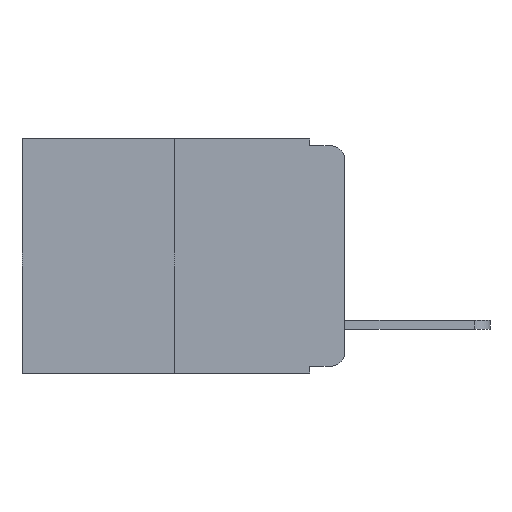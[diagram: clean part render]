
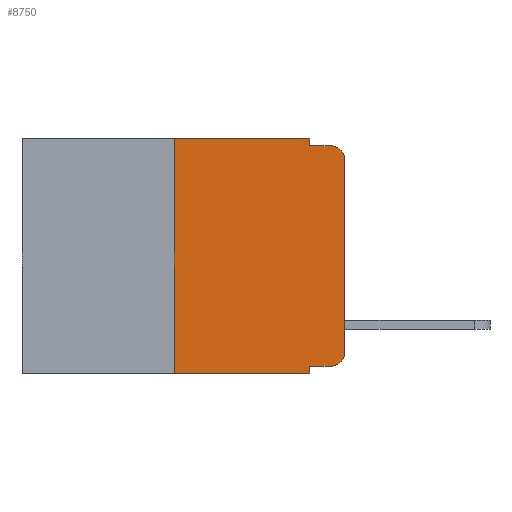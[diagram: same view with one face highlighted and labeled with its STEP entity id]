
A CAD part, left-side view. The second image highlights one B-rep face of the part: STEP entity #8750.
In plain terms, the highlighted planar face has unit normal (-1, 0, 0).
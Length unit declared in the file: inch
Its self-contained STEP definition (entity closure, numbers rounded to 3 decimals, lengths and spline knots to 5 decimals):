
#387 = VECTOR ( 'NONE', #12047, 39.37008 ) ;
#481 = LINE ( 'NONE', #1189, #3764 ) ;
#541 = VERTEX_POINT ( 'NONE', #4985 ) ;
#579 = CARTESIAN_POINT ( 'NONE',  ( 0., 0., 0. ) ) ;
#756 = CARTESIAN_POINT ( 'NONE',  ( 0., 0.051, -0.01 ) ) ;
#1021 = ORIENTED_EDGE ( 'NONE', *, *, #16663, .F. ) ;
#1189 = CARTESIAN_POINT ( 'NONE',  ( 0., 0.051, -0.333 ) ) ;
#1198 = DIRECTION ( 'NONE',  ( 0., -1., 0. ) ) ;
#1387 = VERTEX_POINT ( 'NONE', #7825 ) ;
#1493 = CARTESIAN_POINT ( 'NONE',  ( 0., 0.051, 0. ) ) ;
#1596 = CARTESIAN_POINT ( 'NONE',  ( 0., 0.051, 0. ) ) ;
#2109 = VERTEX_POINT ( 'NONE', #6895 ) ;
#2274 = CARTESIAN_POINT ( 'NONE',  ( 0., 0.25, -0.343 ) ) ;
#2495 = CARTESIAN_POINT ( 'NONE',  ( 0., 0.02, -0.03 ) ) ;
#2586 = EDGE_LOOP ( 'NONE', ( #13434, #10908, #18045, #9063, #1021, #2793, #7592, #9765, #16070, #18382 ) ) ;
#2793 = ORIENTED_EDGE ( 'NONE', *, *, #13953, .F. ) ;
#2866 = EDGE_CURVE ( 'NONE', #5378, #16448, #4866, .T. ) ;
#2891 = LINE ( 'NONE', #6979, #15087 ) ;
#2950 = DIRECTION ( 'NONE',  ( 0., 0., -1. ) ) ;
#3017 = LINE ( 'NONE', #11240, #8993 ) ;
#3072 = VECTOR ( 'NONE', #4361, 39.37008 ) ;
#3764 = VECTOR ( 'NONE', #18364, 39.37008 ) ;
#3909 = DIRECTION ( 'NONE',  ( 0., 0., -1. ) ) ;
#4076 = CARTESIAN_POINT ( 'NONE',  ( 0., 0., -0.03 ) ) ;
#4084 = CARTESIAN_POINT ( 'NONE',  ( 0., 0., -0.313 ) ) ;
#4361 = DIRECTION ( 'NONE',  ( 0., 0., -1. ) ) ;
#4866 = LINE ( 'NONE', #6558, #14208 ) ;
#4965 = VECTOR ( 'NONE', #2950, 39.37008 ) ;
#4985 = CARTESIAN_POINT ( 'NONE',  ( 0., 0.02, -0.333 ) ) ;
#4986 = EDGE_CURVE ( 'NONE', #10221, #15918, #13000, .T. ) ;
#4996 = VERTEX_POINT ( 'NONE', #756 ) ;
#5052 = CARTESIAN_POINT ( 'NONE',  ( 0., 0.25, 0. ) ) ;
#5378 = VERTEX_POINT ( 'NONE', #2274 ) ;
#6446 = CARTESIAN_POINT ( 'NONE',  ( 0., 0.02, -0.01 ) ) ;
#6485 = EDGE_CURVE ( 'NONE', #15918, #8469, #15176, .T. ) ;
#6558 = CARTESIAN_POINT ( 'NONE',  ( 0., 0.473, -0.343 ) ) ;
#6642 = CIRCLE ( 'NONE', #9911, 0.02 ) ;
#6895 = CARTESIAN_POINT ( 'NONE',  ( 0., 0.25, 0. ) ) ;
#6979 = CARTESIAN_POINT ( 'NONE',  ( 0., 0.051, -0.01 ) ) ;
#7115 = DIRECTION ( 'NONE',  ( 0., 0., -1. ) ) ;
#7592 = ORIENTED_EDGE ( 'NONE', *, *, #2866, .T. ) ;
#7825 = CARTESIAN_POINT ( 'NONE',  ( 0., 0.051, -0.333 ) ) ;
#8310 = LINE ( 'NONE', #1493, #4965 ) ;
#8469 = VERTEX_POINT ( 'NONE', #6446 ) ;
#8615 = DIRECTION ( 'NONE',  ( 1., 0., 0. ) ) ;
#8750 = ADVANCED_FACE ( 'NONE', ( #10853 ), #12762, .F. ) ;
#8993 = VECTOR ( 'NONE', #16863, 39.37008 ) ;
#9057 = EDGE_CURVE ( 'NONE', #4996, #8469, #2891, .T. ) ;
#9063 = ORIENTED_EDGE ( 'NONE', *, *, #15511, .F. ) ;
#9162 = DIRECTION ( 'NONE',  ( 0., -1., 0. ) ) ;
#9497 = CARTESIAN_POINT ( 'NONE',  ( 0., 0.051, 0. ) ) ;
#9652 = VERTEX_POINT ( 'NONE', #9497 ) ;
#9695 = LINE ( 'NONE', #1596, #3072 ) ;
#9765 = ORIENTED_EDGE ( 'NONE', *, *, #16818, .F. ) ;
#9911 = AXIS2_PLACEMENT_3D ( 'NONE', #15372, #16880, #15437 ) ;
#10214 = VECTOR ( 'NONE', #13682, 39.37008 ) ;
#10221 = VERTEX_POINT ( 'NONE', #4084 ) ;
#10853 = FACE_OUTER_BOUND ( 'NONE', #2586, .T. ) ;
#10908 = ORIENTED_EDGE ( 'NONE', *, *, #6485, .T. ) ;
#11240 = CARTESIAN_POINT ( 'NONE',  ( 0., 0.473, 0. ) ) ;
#11758 = AXIS2_PLACEMENT_3D ( 'NONE', #16892, #8615, #7115 ) ;
#12047 = DIRECTION ( 'NONE',  ( 0., 0., 1. ) ) ;
#12398 = DIRECTION ( 'NONE',  ( -1., 0., 0. ) ) ;
#12762 = PLANE ( 'NONE',  #11758 ) ;
#13000 = LINE ( 'NONE', #579, #387 ) ;
#13281 = AXIS2_PLACEMENT_3D ( 'NONE', #2495, #12398, #3909 ) ;
#13434 = ORIENTED_EDGE ( 'NONE', *, *, #4986, .T. ) ;
#13662 = CARTESIAN_POINT ( 'NONE',  ( 0., 0.051, -0.343 ) ) ;
#13682 = DIRECTION ( 'NONE',  ( 0., 0., 1. ) ) ;
#13953 = EDGE_CURVE ( 'NONE', #5378, #2109, #14444, .T. ) ;
#14118 = EDGE_CURVE ( 'NONE', #1387, #541, #481, .T. ) ;
#14128 = EDGE_CURVE ( 'NONE', #541, #10221, #6642, .T. ) ;
#14208 = VECTOR ( 'NONE', #9162, 39.37008 ) ;
#14444 = LINE ( 'NONE', #5052, #10214 ) ;
#15087 = VECTOR ( 'NONE', #1198, 39.37008 ) ;
#15176 = CIRCLE ( 'NONE', #13281, 0.02 ) ;
#15372 = CARTESIAN_POINT ( 'NONE',  ( 0., 0.02, -0.313 ) ) ;
#15437 = DIRECTION ( 'NONE',  ( 0., 0., -1. ) ) ;
#15511 = EDGE_CURVE ( 'NONE', #9652, #4996, #9695, .T. ) ;
#15918 = VERTEX_POINT ( 'NONE', #4076 ) ;
#16070 = ORIENTED_EDGE ( 'NONE', *, *, #14118, .T. ) ;
#16448 = VERTEX_POINT ( 'NONE', #13662 ) ;
#16663 = EDGE_CURVE ( 'NONE', #2109, #9652, #3017, .T. ) ;
#16818 = EDGE_CURVE ( 'NONE', #1387, #16448, #8310, .T. ) ;
#16863 = DIRECTION ( 'NONE',  ( 0., -1., 0. ) ) ;
#16880 = DIRECTION ( 'NONE',  ( -1., 0., 0. ) ) ;
#16892 = CARTESIAN_POINT ( 'NONE',  ( 0., 0.473, 0. ) ) ;
#18045 = ORIENTED_EDGE ( 'NONE', *, *, #9057, .F. ) ;
#18364 = DIRECTION ( 'NONE',  ( 0., -1., 0. ) ) ;
#18382 = ORIENTED_EDGE ( 'NONE', *, *, #14128, .T. ) ;
